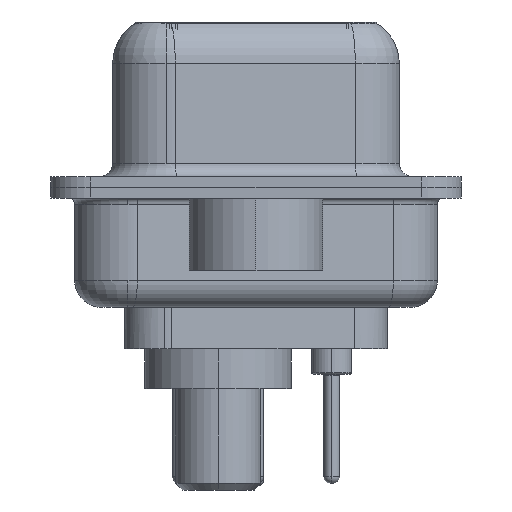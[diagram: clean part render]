
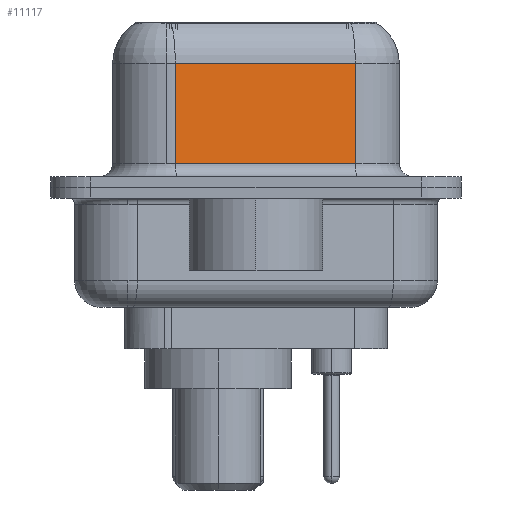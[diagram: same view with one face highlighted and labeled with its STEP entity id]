
A CAD part, left-side view. The second image highlights one B-rep face of the part: STEP entity #11117.
In plain terms, the highlighted planar face has unit normal (-0.985, -0.174, 0).
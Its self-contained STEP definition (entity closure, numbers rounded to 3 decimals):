
#1594 = VECTOR ( 'NONE', #28945, 1000. ) ;
#2685 = ORIENTED_EDGE ( 'NONE', *, *, #2894, .T. ) ;
#2894 = EDGE_CURVE ( 'NONE', #19335, #13331, #3712, .T. ) ;
#3338 = DIRECTION ( 'NONE',  ( 0., 0., -1. ) ) ;
#3712 = LINE ( 'NONE', #11036, #15796 ) ;
#4018 = VERTEX_POINT ( 'NONE', #21713 ) ;
#4218 = DIRECTION ( 'NONE',  ( -0.174, 0.985, 0. ) ) ;
#4593 = DIRECTION ( 'NONE',  ( -0.174, 0.985, 0. ) ) ;
#8363 = CARTESIAN_POINT ( 'NONE',  ( 4.43, 3.028, 0.9 ) ) ;
#8906 = VERTEX_POINT ( 'NONE', #17622 ) ;
#11036 = CARTESIAN_POINT ( 'NONE',  ( 4.43, 3.028, 6.4 ) ) ;
#11117 = ADVANCED_FACE ( 'NONE', ( #12646 ), #12507, .F. ) ;
#11840 = ORIENTED_EDGE ( 'NONE', *, *, #20728, .T. ) ;
#12160 = AXIS2_PLACEMENT_3D ( 'NONE', #33048, #20089, #4593 ) ;
#12229 = VECTOR ( 'NONE', #23476, 1000. ) ;
#12507 = PLANE ( 'NONE',  #12160 ) ;
#12646 = FACE_OUTER_BOUND ( 'NONE', #33129, .T. ) ;
#13331 = VERTEX_POINT ( 'NONE', #8363 ) ;
#13447 = LINE ( 'NONE', #31100, #12229 ) ;
#15796 = VECTOR ( 'NONE', #3338, 1000. ) ;
#16868 = ORIENTED_EDGE ( 'NONE', *, *, #29758, .F. ) ;
#17622 = CARTESIAN_POINT ( 'NONE',  ( 5.621, -3.722, 4.65 ) ) ;
#19335 = VERTEX_POINT ( 'NONE', #28699 ) ;
#19411 = ORIENTED_EDGE ( 'NONE', *, *, #32046, .T. ) ;
#20089 = DIRECTION ( 'NONE',  ( 0.985, 0.174, 0. ) ) ;
#20728 = EDGE_CURVE ( 'NONE', #8906, #19335, #23084, .T. ) ;
#21451 = VECTOR ( 'NONE', #4218, 1000. ) ;
#21713 = CARTESIAN_POINT ( 'NONE',  ( 5.621, -3.722, 0.9 ) ) ;
#22111 = CARTESIAN_POINT ( 'NONE',  ( 5.621, -3.722, 4.65 ) ) ;
#23084 = LINE ( 'NONE', #22111, #21451 ) ;
#23476 = DIRECTION ( 'NONE',  ( 0., 0., -1. ) ) ;
#26579 = CARTESIAN_POINT ( 'NONE',  ( 5.621, -3.722, 0.9 ) ) ;
#28699 = CARTESIAN_POINT ( 'NONE',  ( 4.43, 3.028, 4.65 ) ) ;
#28945 = DIRECTION ( 'NONE',  ( 0.174, -0.985, 0. ) ) ;
#29572 = LINE ( 'NONE', #26579, #1594 ) ;
#29758 = EDGE_CURVE ( 'NONE', #8906, #4018, #13447, .T. ) ;
#31100 = CARTESIAN_POINT ( 'NONE',  ( 5.621, -3.722, 6.4 ) ) ;
#32046 = EDGE_CURVE ( 'NONE', #13331, #4018, #29572, .T. ) ;
#33048 = CARTESIAN_POINT ( 'NONE',  ( 5.621, -3.722, 6.4 ) ) ;
#33129 = EDGE_LOOP ( 'NONE', ( #16868, #11840, #2685, #19411 ) ) ;
